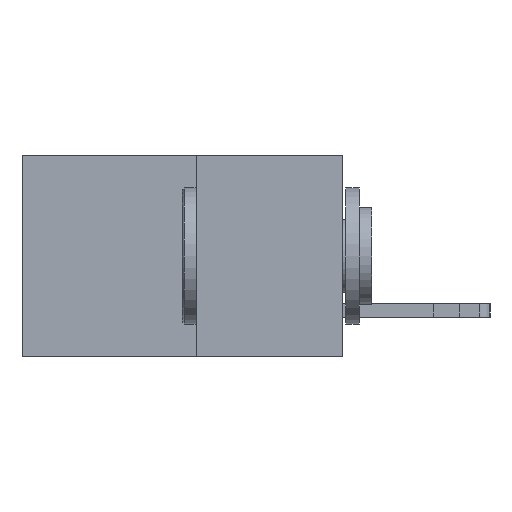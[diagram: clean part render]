
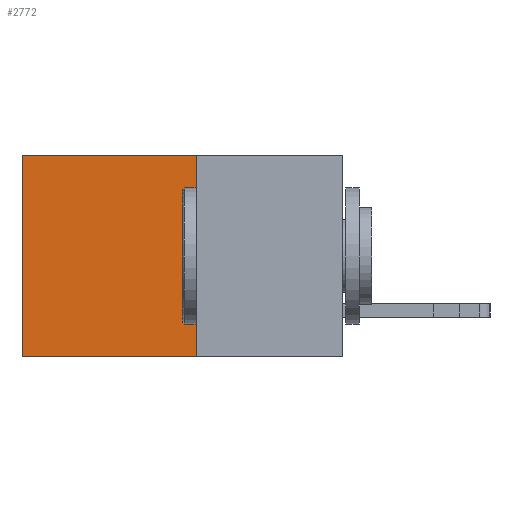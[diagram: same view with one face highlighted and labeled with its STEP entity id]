
A CAD part, left-side view. The second image highlights one B-rep face of the part: STEP entity #2772.
In plain terms, the highlighted planar face has unit normal (-1, 0, 0).
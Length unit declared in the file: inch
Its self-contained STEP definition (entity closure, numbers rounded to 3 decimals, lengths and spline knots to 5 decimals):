
#372 = CARTESIAN_POINT ( 'NONE',  ( 0.277, 0.27, 0. ) ) ;
#418 = EDGE_CURVE ( 'NONE', #18897, #15827, #19867, .T. ) ;
#582 = DIRECTION ( 'NONE',  ( 0., 1., 0. ) ) ;
#1189 = LINE ( 'NONE', #20870, #20752 ) ;
#1804 = CARTESIAN_POINT ( 'NONE',  ( 0.277, 0.59, -0.37 ) ) ;
#2363 = VERTEX_POINT ( 'NONE', #23466 ) ;
#2772 = ADVANCED_FACE ( 'NONE', ( #16946 ), #14453, .F. ) ;
#3889 = ORIENTED_EDGE ( 'NONE', *, *, #21922, .F. ) ;
#5286 = DIRECTION ( 'NONE',  ( 0., 1., 0. ) ) ;
#5408 = ORIENTED_EDGE ( 'NONE', *, *, #10203, .T. ) ;
#6446 = EDGE_LOOP ( 'NONE', ( #5408, #3889, #13921, #15372 ) ) ;
#6760 = LINE ( 'NONE', #1804, #10570 ) ;
#10203 = EDGE_CURVE ( 'NONE', #15827, #11591, #6760, .T. ) ;
#10247 = VECTOR ( 'NONE', #13064, 39.37008 ) ;
#10570 = VECTOR ( 'NONE', #18440, 39.37008 ) ;
#10789 = AXIS2_PLACEMENT_3D ( 'NONE', #14291, #13424, #13376 ) ;
#11591 = VERTEX_POINT ( 'NONE', #14974 ) ;
#13064 = DIRECTION ( 'NONE',  ( 0., 0., -1. ) ) ;
#13376 = DIRECTION ( 'NONE',  ( 0., 0., -1. ) ) ;
#13424 = DIRECTION ( 'NONE',  ( 1., 0., 0. ) ) ;
#13921 = ORIENTED_EDGE ( 'NONE', *, *, #21719, .F. ) ;
#14291 = CARTESIAN_POINT ( 'NONE',  ( 0.277, 0.27, -0.37 ) ) ;
#14453 = PLANE ( 'NONE',  #10789 ) ;
#14974 = CARTESIAN_POINT ( 'NONE',  ( 0.277, 0.59, -0.37 ) ) ;
#15137 = LINE ( 'NONE', #23723, #10247 ) ;
#15372 = ORIENTED_EDGE ( 'NONE', *, *, #418, .T. ) ;
#15827 = VERTEX_POINT ( 'NONE', #23557 ) ;
#16946 = FACE_OUTER_BOUND ( 'NONE', #6446, .T. ) ;
#18440 = DIRECTION ( 'NONE',  ( 0., 0., -1. ) ) ;
#18897 = VERTEX_POINT ( 'NONE', #19338 ) ;
#19313 = VECTOR ( 'NONE', #5286, 39.37008 ) ;
#19338 = CARTESIAN_POINT ( 'NONE',  ( 0.277, 0.27, 0. ) ) ;
#19867 = LINE ( 'NONE', #372, #19313 ) ;
#20752 = VECTOR ( 'NONE', #582, 39.37008 ) ;
#20870 = CARTESIAN_POINT ( 'NONE',  ( 0.277, 0.27, -0.37 ) ) ;
#21719 = EDGE_CURVE ( 'NONE', #18897, #2363, #15137, .T. ) ;
#21922 = EDGE_CURVE ( 'NONE', #2363, #11591, #1189, .T. ) ;
#23466 = CARTESIAN_POINT ( 'NONE',  ( 0.277, 0.27, -0.37 ) ) ;
#23557 = CARTESIAN_POINT ( 'NONE',  ( 0.277, 0.59, 0. ) ) ;
#23723 = CARTESIAN_POINT ( 'NONE',  ( 0.277, 0.27, -0.37 ) ) ;
